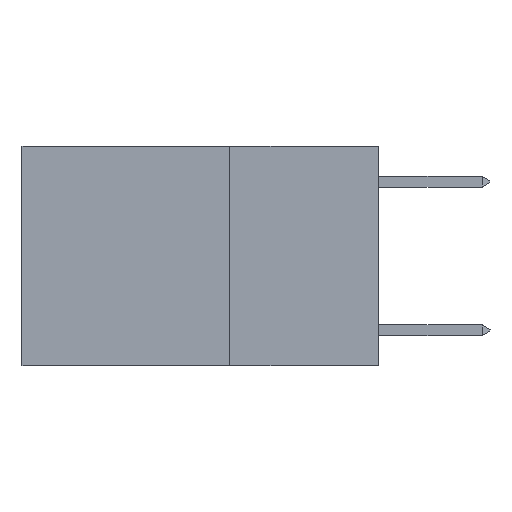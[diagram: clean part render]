
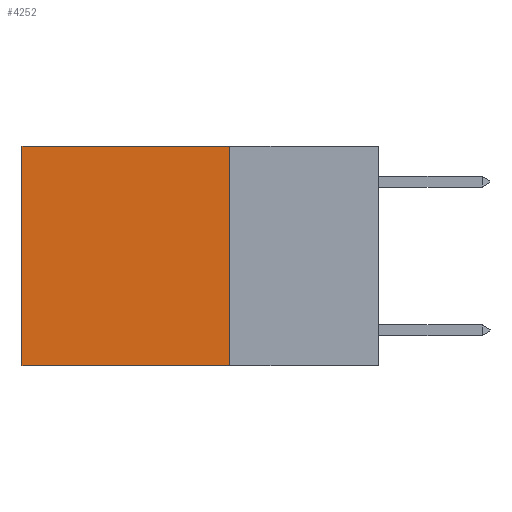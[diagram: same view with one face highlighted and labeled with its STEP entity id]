
A CAD part, left-side view. The second image highlights one B-rep face of the part: STEP entity #4252.
In plain terms, the highlighted planar face has unit normal (-1, 0, 0).
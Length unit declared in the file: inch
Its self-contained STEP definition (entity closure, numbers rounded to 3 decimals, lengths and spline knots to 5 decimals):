
#477 = LINE ( 'NONE', #2892, #7883 ) ;
#687 = PLANE ( 'NONE',  #9125 ) ;
#852 = ORIENTED_EDGE ( 'NONE', *, *, #5737, .F. ) ;
#967 = VECTOR ( 'NONE', #8854, 39.37008 ) ;
#1631 = DIRECTION ( 'NONE',  ( 1., 0., 0. ) ) ;
#1683 = VERTEX_POINT ( 'NONE', #11218 ) ;
#2143 = CARTESIAN_POINT ( 'NONE',  ( 0.2625, 0.6, 0. ) ) ;
#2149 = EDGE_CURVE ( 'NONE', #1683, #8146, #4401, .T. ) ;
#2279 = DIRECTION ( 'NONE',  ( 0., 0., -1. ) ) ;
#2892 = CARTESIAN_POINT ( 'NONE',  ( 0.2625, 0.6, 0. ) ) ;
#3389 = ORIENTED_EDGE ( 'NONE', *, *, #2149, .F. ) ;
#3398 = CARTESIAN_POINT ( 'NONE',  ( 0.2625, 0.25, -0.37 ) ) ;
#4208 = VECTOR ( 'NONE', #9224, 39.37008 ) ;
#4252 = ADVANCED_FACE ( 'NONE', ( #8911 ), #687, .F. ) ;
#4401 = LINE ( 'NONE', #10232, #10951 ) ;
#4563 = EDGE_CURVE ( 'NONE', #1683, #4698, #6307, .T. ) ;
#4698 = VERTEX_POINT ( 'NONE', #2143 ) ;
#5038 = EDGE_CURVE ( 'NONE', #4698, #7417, #477, .T. ) ;
#5737 = EDGE_CURVE ( 'NONE', #8146, #7417, #7458, .T. ) ;
#5773 = CARTESIAN_POINT ( 'NONE',  ( 0.2625, 0.25, -0.37 ) ) ;
#5806 = ORIENTED_EDGE ( 'NONE', *, *, #4563, .T. ) ;
#6307 = LINE ( 'NONE', #7490, #4208 ) ;
#6639 = EDGE_LOOP ( 'NONE', ( #10293, #852, #3389, #5806 ) ) ;
#7200 = CARTESIAN_POINT ( 'NONE',  ( 0.2625, 0.25, 0. ) ) ;
#7417 = VERTEX_POINT ( 'NONE', #8402 ) ;
#7458 = LINE ( 'NONE', #3398, #967 ) ;
#7490 = CARTESIAN_POINT ( 'NONE',  ( 0.2625, 0.25, 0. ) ) ;
#7883 = VECTOR ( 'NONE', #10128, 39.37008 ) ;
#8098 = DIRECTION ( 'NONE',  ( 0., 0., -1. ) ) ;
#8146 = VERTEX_POINT ( 'NONE', #5773 ) ;
#8402 = CARTESIAN_POINT ( 'NONE',  ( 0.2625, 0.6, -0.37 ) ) ;
#8854 = DIRECTION ( 'NONE',  ( 0., 1., 0. ) ) ;
#8911 = FACE_OUTER_BOUND ( 'NONE', #6639, .T. ) ;
#9125 = AXIS2_PLACEMENT_3D ( 'NONE', #7200, #1631, #8098 ) ;
#9224 = DIRECTION ( 'NONE',  ( 0., 1., 0. ) ) ;
#10128 = DIRECTION ( 'NONE',  ( 0., 0., -1. ) ) ;
#10232 = CARTESIAN_POINT ( 'NONE',  ( 0.2625, 0.25, 0. ) ) ;
#10293 = ORIENTED_EDGE ( 'NONE', *, *, #5038, .T. ) ;
#10951 = VECTOR ( 'NONE', #2279, 39.37008 ) ;
#11218 = CARTESIAN_POINT ( 'NONE',  ( 0.2625, 0.25, 0. ) ) ;
